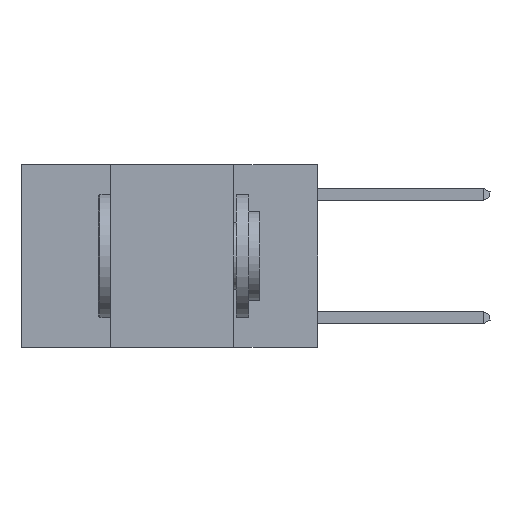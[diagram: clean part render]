
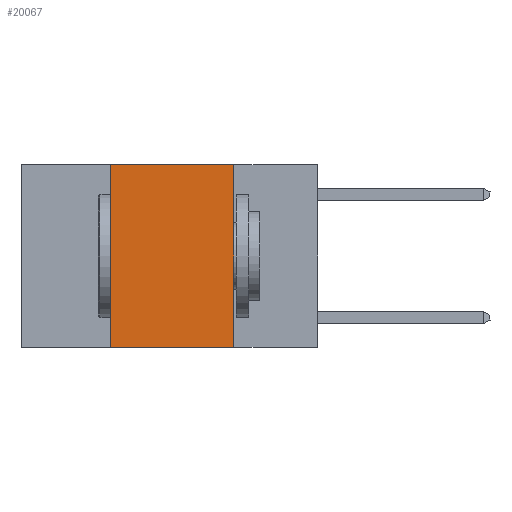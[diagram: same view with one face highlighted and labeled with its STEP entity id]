
A CAD part, left-side view. The second image highlights one B-rep face of the part: STEP entity #20067.
In plain terms, the highlighted planar face has unit normal (-1, 0, 0).
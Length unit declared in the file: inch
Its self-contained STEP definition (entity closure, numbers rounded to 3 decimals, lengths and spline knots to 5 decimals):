
#500 = LINE ( 'NONE', #5155, #18270 ) ;
#1130 = VERTEX_POINT ( 'NONE', #14824 ) ;
#1667 = DIRECTION ( 'NONE',  ( 0., 0., -1. ) ) ;
#1881 = CARTESIAN_POINT ( 'NONE',  ( 0., 0.17, 0. ) ) ;
#1976 = FACE_OUTER_BOUND ( 'NONE', #10493, .T. ) ;
#2462 = CARTESIAN_POINT ( 'NONE',  ( 0., 0.6, 0. ) ) ;
#2576 = DIRECTION ( 'NONE',  ( 0., -1., 0. ) ) ;
#3364 = DIRECTION ( 'NONE',  ( 1., 0., 0. ) ) ;
#4129 = CARTESIAN_POINT ( 'NONE',  ( 0., 0.42, 0. ) ) ;
#4944 = PLANE ( 'NONE',  #16392 ) ;
#4953 = DIRECTION ( 'NONE',  ( 0., 0., -1. ) ) ;
#5155 = CARTESIAN_POINT ( 'NONE',  ( 0., 0.42, 0. ) ) ;
#6558 = CARTESIAN_POINT ( 'NONE',  ( 0., 0.42, -0.37 ) ) ;
#7005 = EDGE_CURVE ( 'NONE', #14987, #1130, #9271, .T. ) ;
#7075 = DIRECTION ( 'NONE',  ( 0., 0., 1. ) ) ;
#7533 = CARTESIAN_POINT ( 'NONE',  ( 0., 0.6, -0.37 ) ) ;
#9271 = LINE ( 'NONE', #7533, #13650 ) ;
#9831 = LINE ( 'NONE', #1881, #14319 ) ;
#10493 = EDGE_LOOP ( 'NONE', ( #12365, #20006, #13036, #15907 ) ) ;
#11006 = EDGE_CURVE ( 'NONE', #14733, #14717, #17045, .T. ) ;
#11439 = CARTESIAN_POINT ( 'NONE',  ( 0., 0.6, 0. ) ) ;
#12365 = ORIENTED_EDGE ( 'NONE', *, *, #17330, .F. ) ;
#13036 = ORIENTED_EDGE ( 'NONE', *, *, #13132, .F. ) ;
#13106 = VECTOR ( 'NONE', #2576, 39.37008 ) ;
#13132 = EDGE_CURVE ( 'NONE', #14987, #14733, #500, .T. ) ;
#13650 = VECTOR ( 'NONE', #20531, 39.37008 ) ;
#14319 = VECTOR ( 'NONE', #4953, 39.37008 ) ;
#14717 = VERTEX_POINT ( 'NONE', #20091 ) ;
#14733 = VERTEX_POINT ( 'NONE', #4129 ) ;
#14824 = CARTESIAN_POINT ( 'NONE',  ( 0., 0.17, -0.37 ) ) ;
#14987 = VERTEX_POINT ( 'NONE', #6558 ) ;
#15907 = ORIENTED_EDGE ( 'NONE', *, *, #7005, .T. ) ;
#16392 = AXIS2_PLACEMENT_3D ( 'NONE', #11439, #3364, #1667 ) ;
#17045 = LINE ( 'NONE', #2462, #13106 ) ;
#17330 = EDGE_CURVE ( 'NONE', #14717, #1130, #9831, .T. ) ;
#18270 = VECTOR ( 'NONE', #7075, 39.37008 ) ;
#20006 = ORIENTED_EDGE ( 'NONE', *, *, #11006, .F. ) ;
#20067 = ADVANCED_FACE ( 'NONE', ( #1976 ), #4944, .F. ) ;
#20091 = CARTESIAN_POINT ( 'NONE',  ( 0., 0.17, 0. ) ) ;
#20531 = DIRECTION ( 'NONE',  ( 0., -1., 0. ) ) ;
